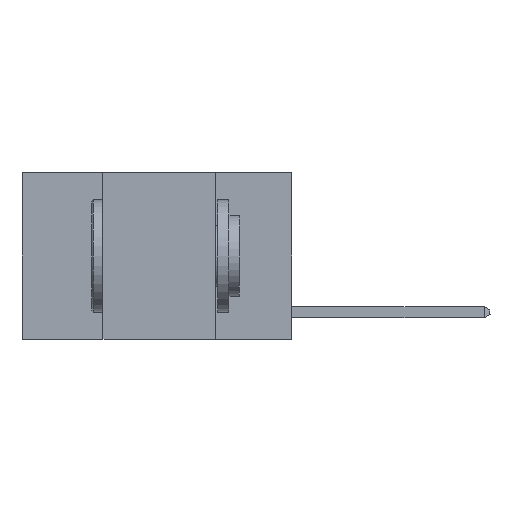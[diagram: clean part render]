
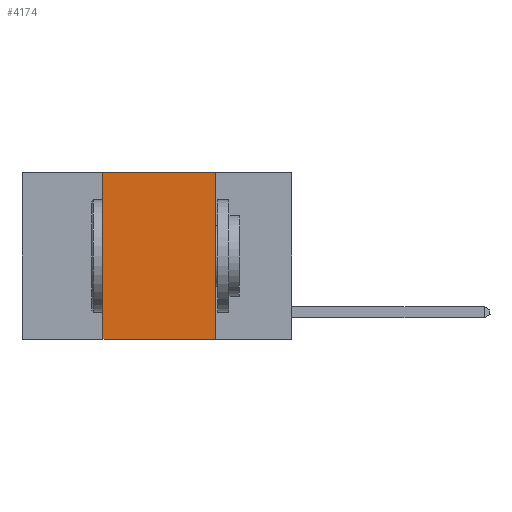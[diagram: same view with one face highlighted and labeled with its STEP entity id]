
A CAD part, left-side view. The second image highlights one B-rep face of the part: STEP entity #4174.
In plain terms, the highlighted planar face has unit normal (-1, 0, 0).
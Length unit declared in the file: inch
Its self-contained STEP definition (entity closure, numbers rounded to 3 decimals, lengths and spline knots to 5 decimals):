
#30 = EDGE_LOOP ( 'NONE', ( #2879, #5315, #1578, #3772 ) ) ;
#846 = CARTESIAN_POINT ( 'NONE',  ( 0., 0.42, 0. ) ) ;
#973 = CARTESIAN_POINT ( 'NONE',  ( 0., 0.6, 0. ) ) ;
#1103 = VECTOR ( 'NONE', #1296, 39.37008 ) ;
#1264 = LINE ( 'NONE', #6525, #1631 ) ;
#1296 = DIRECTION ( 'NONE',  ( 0., 0., 1. ) ) ;
#1578 = ORIENTED_EDGE ( 'NONE', *, *, #3767, .F. ) ;
#1631 = VECTOR ( 'NONE', #3663, 39.37008 ) ;
#1851 = DIRECTION ( 'NONE',  ( 0., 0., -1. ) ) ;
#2085 = VERTEX_POINT ( 'NONE', #9132 ) ;
#2094 = CARTESIAN_POINT ( 'NONE',  ( 0., 0.42, 0. ) ) ;
#2482 = DIRECTION ( 'NONE',  ( 0., -1., 0. ) ) ;
#2879 = ORIENTED_EDGE ( 'NONE', *, *, #7341, .F. ) ;
#3663 = DIRECTION ( 'NONE',  ( 0., 0., -1. ) ) ;
#3767 = EDGE_CURVE ( 'NONE', #8439, #8837, #8879, .T. ) ;
#3772 = ORIENTED_EDGE ( 'NONE', *, *, #7644, .T. ) ;
#4174 = ADVANCED_FACE ( 'NONE', ( #9727 ), #4731, .F. ) ;
#4177 = CARTESIAN_POINT ( 'NONE',  ( 0., 0.42, -0.37 ) ) ;
#4731 = PLANE ( 'NONE',  #7941 ) ;
#5315 = ORIENTED_EDGE ( 'NONE', *, *, #7612, .F. ) ;
#5414 = VECTOR ( 'NONE', #2482, 39.37008 ) ;
#6248 = DIRECTION ( 'NONE',  ( 1., 0., 0. ) ) ;
#6525 = CARTESIAN_POINT ( 'NONE',  ( 0., 0.17, 0. ) ) ;
#6888 = LINE ( 'NONE', #6941, #5414 ) ;
#6941 = CARTESIAN_POINT ( 'NONE',  ( 0., 0.6, 0. ) ) ;
#7341 = EDGE_CURVE ( 'NONE', #2085, #8479, #1264, .T. ) ;
#7612 = EDGE_CURVE ( 'NONE', #8837, #2085, #6888, .T. ) ;
#7644 = EDGE_CURVE ( 'NONE', #8439, #8479, #8217, .T. ) ;
#7941 = AXIS2_PLACEMENT_3D ( 'NONE', #973, #6248, #1851 ) ;
#8217 = LINE ( 'NONE', #9656, #9202 ) ;
#8439 = VERTEX_POINT ( 'NONE', #4177 ) ;
#8479 = VERTEX_POINT ( 'NONE', #9558 ) ;
#8837 = VERTEX_POINT ( 'NONE', #846 ) ;
#8879 = LINE ( 'NONE', #2094, #1103 ) ;
#9132 = CARTESIAN_POINT ( 'NONE',  ( 0., 0.17, 0. ) ) ;
#9202 = VECTOR ( 'NONE', #9705, 39.37008 ) ;
#9558 = CARTESIAN_POINT ( 'NONE',  ( 0., 0.17, -0.37 ) ) ;
#9656 = CARTESIAN_POINT ( 'NONE',  ( 0., 0.6, -0.37 ) ) ;
#9705 = DIRECTION ( 'NONE',  ( 0., -1., 0. ) ) ;
#9727 = FACE_OUTER_BOUND ( 'NONE', #30, .T. ) ;
